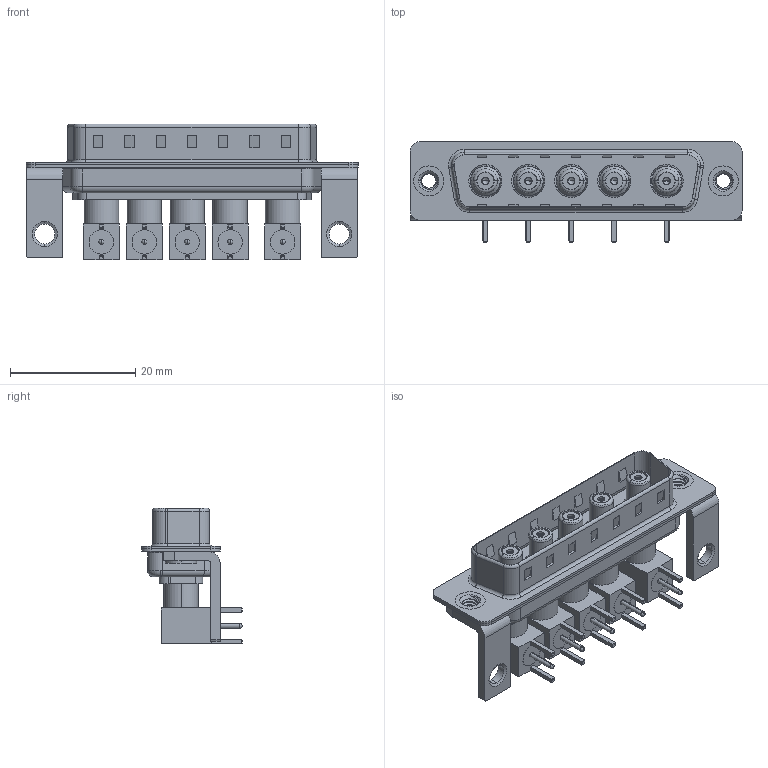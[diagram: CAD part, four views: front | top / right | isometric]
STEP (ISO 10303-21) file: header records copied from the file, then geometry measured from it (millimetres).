
FILE_DESCRIPTION (( 'STEP AP203' ), '1' );
FILE_NAME ('629-5W5-240-5T4.STEP', '2022-05-07T05:51:59', ( '' ), ( '' ), 'SwSTEP 2.0', 'SolidWorks 2020', '' );
FILE_SCHEMA (( 'CONFIG_CONTROL_DESIGN' ));
Length unit declared in the file: millimetre
Products named in the file (18): Co-Ax Jack_RA PC Tail; Locking Collar; Co-Ax Jack Assy_RA; 629Combo Housing_5W5; 629Combo Threaded Rivet_3; 629-5W5-240-5T4; RA Back Shell; Insulator Socket; Insulator RA Pin; 629Combo Shell Rear_25 Contacts; Socket_RA; 629Combo Shell Front_25 Contacts; Insulator Socket 2; 629Combo Stabilizer Bracket
Assembly tree (47 placements, depth 3):
  629-5W5-240-5T4
    629Combo Housing_5W5
    629Combo Shell Rear_25 Contacts
    629Combo Shell Front_25 Contacts
    629Combo Threaded Rivet_3  x2
    629Combo Stabilizer Bracket  x2
    Co-Ax Jack Assy_RA
      Co-Ax Jack_RA PC Tail
      Insulator Socket
      Insulator Socket 2
      Locking Collar
      Socket_RA
      RA Back Shell
      Insulator RA Pin
    Co-Ax Jack Assy_RA
      Co-Ax Jack_RA PC Tail
      Insulator Socket
      Insulator Socket 2
      Locking Collar
      Socket_RA
      RA Back Shell
      Insulator RA Pin
    Co-Ax Jack Assy_RA
      Co-Ax Jack_RA PC Tail
      Insulator Socket
      Insulator Socket 2
      Locking Collar
      Socket_RA
      RA Back Shell
      Insulator RA Pin
    Co-Ax Jack Assy_RA
      Co-Ax Jack_RA PC Tail
      Insulator Socket
      Insulator Socket 2
      Locking Collar
      Socket_RA
      RA Back Shell
      Insulator RA Pin
    Co-Ax Jack Assy_RA
      Co-Ax Jack_RA PC Tail
      Insulator Socket
      Insulator Socket 2
      Locking Collar
      Socket_RA
      RA Back Shell
      Insulator RA Pin
Bounding box: 53.05 x 16 x 21.71 mm (x, y, z)
Volume: 4411.2 mm3; surface area: 11955.5 mm2
Topology: 42 solids, 42 shells, 1176 faces, 2788 edges, 1737 vertices
Faces by surface type: cylinder 490, plane 476, cone 109, torus 80, bspline 11, sphere 10
Entity records: 20289 total; most frequent: CARTESIAN_POINT 4391, DIRECTION 2930, ORIENTED_EDGE 2620, EDGE_CURVE 1310, AXIS2_PLACEMENT_3D 1093, VERTEX_POINT 828, LINE 744, VECTOR 744
